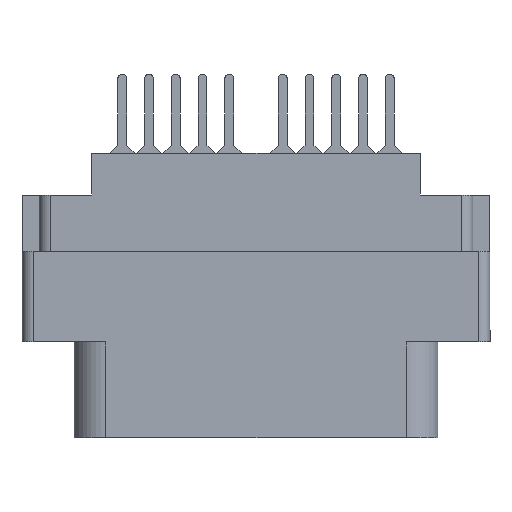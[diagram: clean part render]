
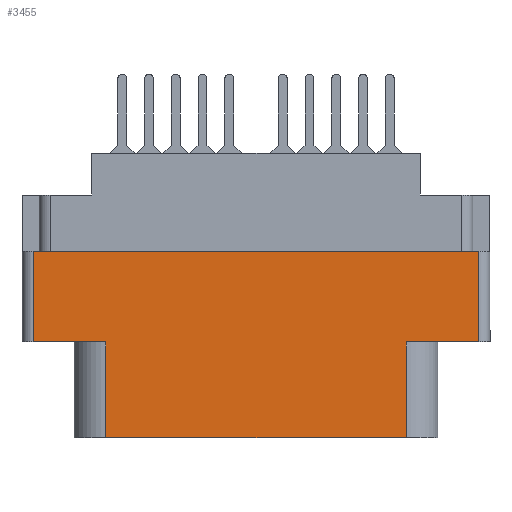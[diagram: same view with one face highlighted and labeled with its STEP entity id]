
A CAD part, front view. The second image highlights one B-rep face of the part: STEP entity #3455.
In plain terms, the highlighted planar face has unit normal (0, -1, 0).
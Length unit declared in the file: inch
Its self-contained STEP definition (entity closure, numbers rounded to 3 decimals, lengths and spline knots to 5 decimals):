
#120 = ORIENTED_EDGE ( 'NONE', *, *, #18319, .T. ) ;
#145 = VERTEX_POINT ( 'NONE', #11185 ) ;
#702 = FACE_OUTER_BOUND ( 'NONE', #20218, .T. ) ;
#1020 = EDGE_CURVE ( 'NONE', #12039, #19738, #6987, .T. ) ;
#1144 = ORIENTED_EDGE ( 'NONE', *, *, #9035, .F. ) ;
#1750 = LINE ( 'NONE', #20792, #7553 ) ;
#2487 = VECTOR ( 'NONE', #8411, 39.37008 ) ;
#2867 = CARTESIAN_POINT ( 'NONE',  ( -0.624, -0.343, -0.529 ) ) ;
#2981 = DIRECTION ( 'NONE',  ( 1., 0., 0. ) ) ;
#3455 = ADVANCED_FACE ( 'NONE', ( #702 ), #17576, .T. ) ;
#4456 = CARTESIAN_POINT ( 'NONE',  ( -0.42052, -0.343, -0.529 ) ) ;
#4466 = CARTESIAN_POINT ( 'NONE',  ( -0.42052, -0.343, -0.798 ) ) ;
#5591 = ORIENTED_EDGE ( 'NONE', *, *, #10968, .T. ) ;
#6825 = LINE ( 'NONE', #18554, #11161 ) ;
#6987 = LINE ( 'NONE', #11459, #20527 ) ;
#7012 = VERTEX_POINT ( 'NONE', #4466 ) ;
#7553 = VECTOR ( 'NONE', #13472, 39.37008 ) ;
#7955 = LINE ( 'NONE', #22606, #11427 ) ;
#8071 = CARTESIAN_POINT ( 'NONE',  ( -0.656, -0.343, -0.798 ) ) ;
#8336 = CARTESIAN_POINT ( 'NONE',  ( 0.42052, -0.343, -0.798 ) ) ;
#8411 = DIRECTION ( 'NONE',  ( 0., 0., 1. ) ) ;
#8749 = CARTESIAN_POINT ( 'NONE',  ( 0.42052, -0.343, -0.529 ) ) ;
#9014 = DIRECTION ( 'NONE',  ( 1., 0., 0. ) ) ;
#9035 = EDGE_CURVE ( 'NONE', #15874, #20989, #22394, .T. ) ;
#9601 = DIRECTION ( 'NONE',  ( -1., 0., 0. ) ) ;
#10028 = DIRECTION ( 'NONE',  ( 0., 0., -1. ) ) ;
#10459 = CARTESIAN_POINT ( 'NONE',  ( 0.624, -0.343, -0.274 ) ) ;
#10894 = DIRECTION ( 'NONE',  ( 0., 0., 1. ) ) ;
#10968 = EDGE_CURVE ( 'NONE', #7012, #19285, #16444, .T. ) ;
#11161 = VECTOR ( 'NONE', #10894, 39.37008 ) ;
#11185 = CARTESIAN_POINT ( 'NONE',  ( 0.42052, -0.343, -0.529 ) ) ;
#11306 = DIRECTION ( 'NONE',  ( 1., 0., 0. ) ) ;
#11427 = VECTOR ( 'NONE', #22763, 39.37008 ) ;
#11459 = CARTESIAN_POINT ( 'NONE',  ( 0., -0.343, -0.529 ) ) ;
#12039 = VERTEX_POINT ( 'NONE', #2867 ) ;
#12662 = VERTEX_POINT ( 'NONE', #13973 ) ;
#12679 = ORIENTED_EDGE ( 'NONE', *, *, #16275, .F. ) ;
#12751 = EDGE_CURVE ( 'NONE', #19285, #145, #12927, .T. ) ;
#12927 = LINE ( 'NONE', #8749, #2487 ) ;
#13395 = CARTESIAN_POINT ( 'NONE',  ( -0.624, -0.343, -0.274 ) ) ;
#13472 = DIRECTION ( 'NONE',  ( 0., 0., -1. ) ) ;
#13667 = EDGE_CURVE ( 'NONE', #15874, #12039, #7955, .T. ) ;
#13973 = CARTESIAN_POINT ( 'NONE',  ( 0.624, -0.343, -0.529 ) ) ;
#14921 = VECTOR ( 'NONE', #9014, 39.37008 ) ;
#15862 = VECTOR ( 'NONE', #9601, 39.37008 ) ;
#15874 = VERTEX_POINT ( 'NONE', #13395 ) ;
#16196 = ORIENTED_EDGE ( 'NONE', *, *, #21708, .T. ) ;
#16275 = EDGE_CURVE ( 'NONE', #12662, #145, #17906, .T. ) ;
#16444 = LINE ( 'NONE', #21591, #19035 ) ;
#17489 = DIRECTION ( 'NONE',  ( 0., -1., 0. ) ) ;
#17576 = PLANE ( 'NONE',  #22534 ) ;
#17906 = LINE ( 'NONE', #20612, #15862 ) ;
#18017 = ORIENTED_EDGE ( 'NONE', *, *, #1020, .T. ) ;
#18319 = EDGE_CURVE ( 'NONE', #12662, #20989, #6825, .T. ) ;
#18554 = CARTESIAN_POINT ( 'NONE',  ( 0.624, -0.343, -0.798 ) ) ;
#19035 = VECTOR ( 'NONE', #2981, 39.37008 ) ;
#19285 = VERTEX_POINT ( 'NONE', #8336 ) ;
#19738 = VERTEX_POINT ( 'NONE', #4456 ) ;
#20218 = EDGE_LOOP ( 'NONE', ( #1144, #21024, #18017, #16196, #5591, #21057, #12679, #120 ) ) ;
#20527 = VECTOR ( 'NONE', #11306, 39.37008 ) ;
#20612 = CARTESIAN_POINT ( 'NONE',  ( 0., -0.343, -0.529 ) ) ;
#20792 = CARTESIAN_POINT ( 'NONE',  ( -0.42052, -0.343, -0.798 ) ) ;
#20989 = VERTEX_POINT ( 'NONE', #10459 ) ;
#21024 = ORIENTED_EDGE ( 'NONE', *, *, #13667, .T. ) ;
#21057 = ORIENTED_EDGE ( 'NONE', *, *, #12751, .T. ) ;
#21591 = CARTESIAN_POINT ( 'NONE',  ( -0.656, -0.343, -0.798 ) ) ;
#21708 = EDGE_CURVE ( 'NONE', #19738, #7012, #1750, .T. ) ;
#21935 = CARTESIAN_POINT ( 'NONE',  ( 0., -0.343, -0.274 ) ) ;
#22394 = LINE ( 'NONE', #21935, #14921 ) ;
#22534 = AXIS2_PLACEMENT_3D ( 'NONE', #8071, #17489, #10028 ) ;
#22606 = CARTESIAN_POINT ( 'NONE',  ( -0.624, -0.343, -0.798 ) ) ;
#22763 = DIRECTION ( 'NONE',  ( 0., 0., -1. ) ) ;
